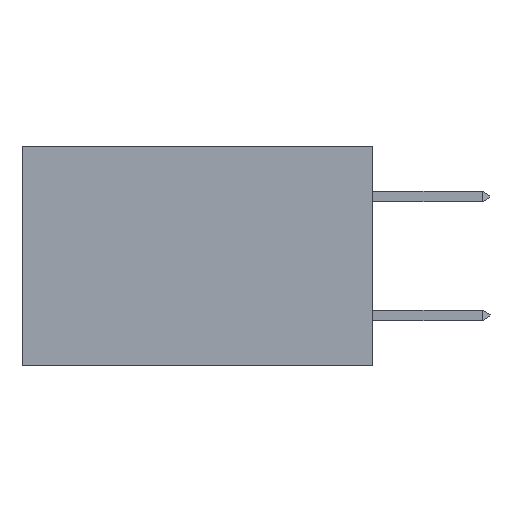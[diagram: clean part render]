
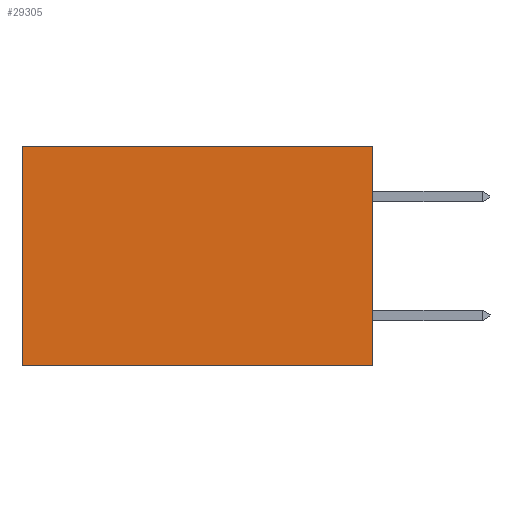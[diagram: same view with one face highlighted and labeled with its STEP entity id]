
A CAD part, left-side view. The second image highlights one B-rep face of the part: STEP entity #29305.
In plain terms, the highlighted planar face has unit normal (-1, 0, 0).
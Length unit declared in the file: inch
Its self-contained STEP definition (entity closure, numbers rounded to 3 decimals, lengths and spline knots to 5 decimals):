
#1794 = VECTOR ( 'NONE', #5345, 39.37008 ) ;
#2158 = VECTOR ( 'NONE', #31823, 39.37008 ) ;
#2251 = LINE ( 'NONE', #28233, #21904 ) ;
#2585 = LINE ( 'NONE', #22519, #1794 ) ;
#2666 = CARTESIAN_POINT ( 'NONE',  ( 0.277, 0., -0.37 ) ) ;
#3743 = ORIENTED_EDGE ( 'NONE', *, *, #21630, .F. ) ;
#4331 = ORIENTED_EDGE ( 'NONE', *, *, #22263, .T. ) ;
#4724 = VERTEX_POINT ( 'NONE', #7708 ) ;
#5345 = DIRECTION ( 'NONE',  ( 0., 1., 0. ) ) ;
#5871 = CARTESIAN_POINT ( 'NONE',  ( 0.277, 0., -0.37 ) ) ;
#7000 = VECTOR ( 'NONE', #28045, 39.37008 ) ;
#7708 = CARTESIAN_POINT ( 'NONE',  ( 0.277, 0.59, -0.37 ) ) ;
#12026 = VERTEX_POINT ( 'NONE', #17972 ) ;
#12527 = VERTEX_POINT ( 'NONE', #2666 ) ;
#14197 = AXIS2_PLACEMENT_3D ( 'NONE', #18225, #30651, #15882 ) ;
#14542 = LINE ( 'NONE', #29410, #2158 ) ;
#15057 = LINE ( 'NONE', #5871, #7000 ) ;
#15882 = DIRECTION ( 'NONE',  ( 0., 0., -1. ) ) ;
#15916 = DIRECTION ( 'NONE',  ( 0., 1., 0. ) ) ;
#15935 = VERTEX_POINT ( 'NONE', #27730 ) ;
#17972 = CARTESIAN_POINT ( 'NONE',  ( 0.277, 0., 0. ) ) ;
#18225 = CARTESIAN_POINT ( 'NONE',  ( 0.277, 0., -0.37 ) ) ;
#19304 = EDGE_LOOP ( 'NONE', ( #30569, #23820, #3743, #4331 ) ) ;
#20700 = PLANE ( 'NONE',  #14197 ) ;
#21630 = EDGE_CURVE ( 'NONE', #12026, #12527, #15057, .T. ) ;
#21904 = VECTOR ( 'NONE', #15916, 39.37008 ) ;
#22263 = EDGE_CURVE ( 'NONE', #12026, #15935, #2251, .T. ) ;
#22519 = CARTESIAN_POINT ( 'NONE',  ( 0.277, 0., -0.37 ) ) ;
#23642 = EDGE_CURVE ( 'NONE', #15935, #4724, #14542, .T. ) ;
#23820 = ORIENTED_EDGE ( 'NONE', *, *, #29800, .F. ) ;
#27730 = CARTESIAN_POINT ( 'NONE',  ( 0.277, 0.59, 0. ) ) ;
#28045 = DIRECTION ( 'NONE',  ( 0., 0., -1. ) ) ;
#28233 = CARTESIAN_POINT ( 'NONE',  ( 0.277, 0., 0. ) ) ;
#29305 = ADVANCED_FACE ( 'NONE', ( #29634 ), #20700, .F. ) ;
#29410 = CARTESIAN_POINT ( 'NONE',  ( 0.277, 0.59, -0.37 ) ) ;
#29634 = FACE_OUTER_BOUND ( 'NONE', #19304, .T. ) ;
#29800 = EDGE_CURVE ( 'NONE', #12527, #4724, #2585, .T. ) ;
#30569 = ORIENTED_EDGE ( 'NONE', *, *, #23642, .T. ) ;
#30651 = DIRECTION ( 'NONE',  ( 1., 0., 0. ) ) ;
#31823 = DIRECTION ( 'NONE',  ( 0., 0., -1. ) ) ;
